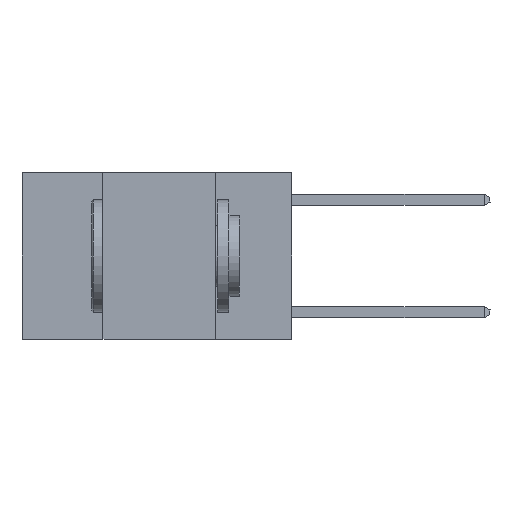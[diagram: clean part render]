
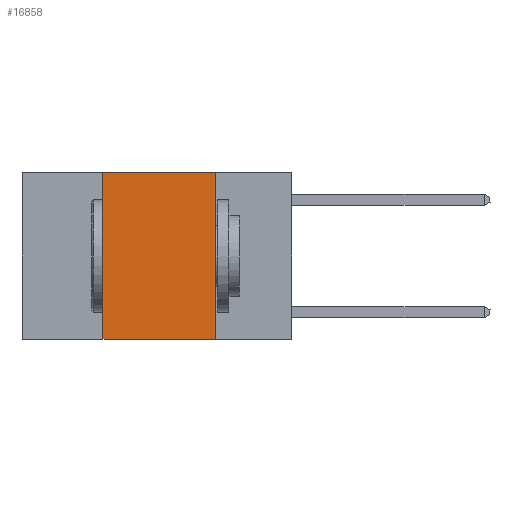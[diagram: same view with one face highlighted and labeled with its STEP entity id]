
A CAD part, left-side view. The second image highlights one B-rep face of the part: STEP entity #16858.
In plain terms, the highlighted planar face has unit normal (-1, 0, 0).
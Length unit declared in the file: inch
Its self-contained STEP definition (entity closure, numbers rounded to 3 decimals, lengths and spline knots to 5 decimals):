
#12 = VECTOR ( 'NONE', #26443, 39.37008 ) ;
#302 = ORIENTED_EDGE ( 'NONE', *, *, #15217, .T. ) ;
#398 = LINE ( 'NONE', #7266, #24005 ) ;
#2654 = LINE ( 'NONE', #26594, #12 ) ;
#3040 = ORIENTED_EDGE ( 'NONE', *, *, #28406, .F. ) ;
#3401 = ORIENTED_EDGE ( 'NONE', *, *, #8545, .F. ) ;
#3583 = CARTESIAN_POINT ( 'NONE',  ( 0., 0.42, 0. ) ) ;
#4447 = DIRECTION ( 'NONE',  ( 0., 0., -1. ) ) ;
#7266 = CARTESIAN_POINT ( 'NONE',  ( 0., 0.6, 0. ) ) ;
#8180 = EDGE_CURVE ( 'NONE', #28533, #26569, #398, .T. ) ;
#8250 = DIRECTION ( 'NONE',  ( 0., 0., 1. ) ) ;
#8545 = EDGE_CURVE ( 'NONE', #13776, #28533, #27080, .T. ) ;
#9814 = CARTESIAN_POINT ( 'NONE',  ( 0., 0.6, -0.37 ) ) ;
#11822 = VECTOR ( 'NONE', #18835, 39.37008 ) ;
#12376 = AXIS2_PLACEMENT_3D ( 'NONE', #15771, #28202, #4447 ) ;
#13776 = VERTEX_POINT ( 'NONE', #22041 ) ;
#14952 = CARTESIAN_POINT ( 'NONE',  ( 0., 0.17, 0. ) ) ;
#15217 = EDGE_CURVE ( 'NONE', #13776, #29863, #23967, .T. ) ;
#15402 = CARTESIAN_POINT ( 'NONE',  ( 0., 0.42, 0. ) ) ;
#15771 = CARTESIAN_POINT ( 'NONE',  ( 0., 0.6, 0. ) ) ;
#16858 = ADVANCED_FACE ( 'NONE', ( #18080 ), #30558, .F. ) ;
#17371 = EDGE_LOOP ( 'NONE', ( #3040, #25488, #3401, #302 ) ) ;
#18080 = FACE_OUTER_BOUND ( 'NONE', #17371, .T. ) ;
#18835 = DIRECTION ( 'NONE',  ( 0., -1., 0. ) ) ;
#19361 = DIRECTION ( 'NONE',  ( 0., -1., 0. ) ) ;
#21673 = CARTESIAN_POINT ( 'NONE',  ( 0., 0.17, -0.37 ) ) ;
#22041 = CARTESIAN_POINT ( 'NONE',  ( 0., 0.42, -0.37 ) ) ;
#23030 = VECTOR ( 'NONE', #8250, 39.37008 ) ;
#23967 = LINE ( 'NONE', #9814, #11822 ) ;
#24005 = VECTOR ( 'NONE', #19361, 39.37008 ) ;
#25488 = ORIENTED_EDGE ( 'NONE', *, *, #8180, .F. ) ;
#26443 = DIRECTION ( 'NONE',  ( 0., 0., -1. ) ) ;
#26569 = VERTEX_POINT ( 'NONE', #14952 ) ;
#26594 = CARTESIAN_POINT ( 'NONE',  ( 0., 0.17, 0. ) ) ;
#27080 = LINE ( 'NONE', #15402, #23030 ) ;
#28202 = DIRECTION ( 'NONE',  ( 1., 0., 0. ) ) ;
#28406 = EDGE_CURVE ( 'NONE', #26569, #29863, #2654, .T. ) ;
#28533 = VERTEX_POINT ( 'NONE', #3583 ) ;
#29863 = VERTEX_POINT ( 'NONE', #21673 ) ;
#30558 = PLANE ( 'NONE',  #12376 ) ;
